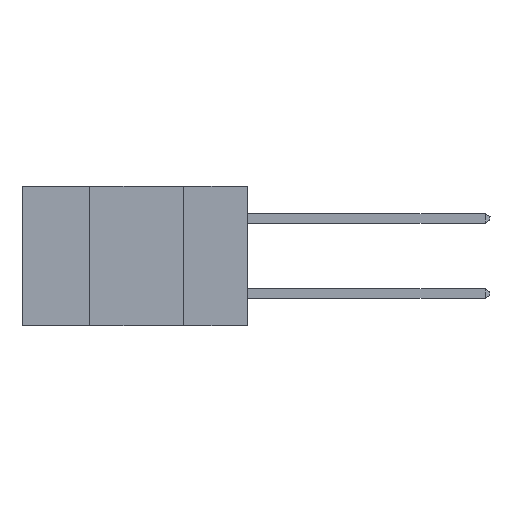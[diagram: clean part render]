
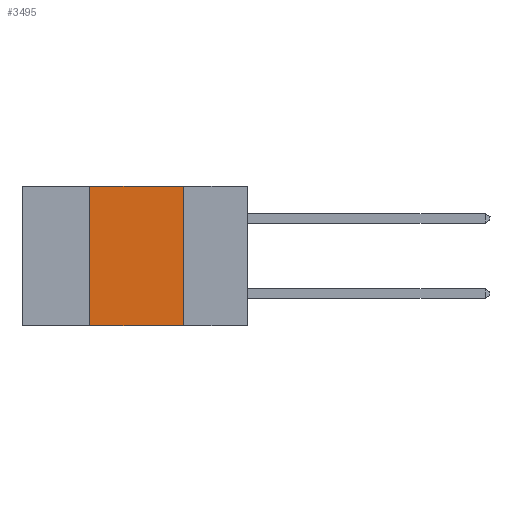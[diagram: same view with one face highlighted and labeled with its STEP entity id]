
A CAD part, left-side view. The second image highlights one B-rep face of the part: STEP entity #3495.
In plain terms, the highlighted planar face has unit normal (-1, 0, 0).
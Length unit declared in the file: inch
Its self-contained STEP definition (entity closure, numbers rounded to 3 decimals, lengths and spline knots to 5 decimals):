
#65 = DIRECTION ( 'NONE',  ( 0., -1., 0. ) ) ;
#738 = DIRECTION ( 'NONE',  ( 0., -1., 0. ) ) ;
#1065 = EDGE_CURVE ( 'NONE', #9933, #8915, #4147, .T. ) ;
#1200 = ORIENTED_EDGE ( 'NONE', *, *, #1065, .F. ) ;
#2044 = VERTEX_POINT ( 'NONE', #11692 ) ;
#2107 = DIRECTION ( 'NONE',  ( 0., 0., -1. ) ) ;
#2259 = DIRECTION ( 'NONE',  ( 0., 0., 1. ) ) ;
#2519 = LINE ( 'NONE', #5392, #11917 ) ;
#2683 = ORIENTED_EDGE ( 'NONE', *, *, #5785, .F. ) ;
#2806 = PLANE ( 'NONE',  #11710 ) ;
#3495 = ADVANCED_FACE ( 'NONE', ( #6768 ), #2806, .F. ) ;
#3760 = CARTESIAN_POINT ( 'NONE',  ( 0., 0.6, 0. ) ) ;
#3785 = LINE ( 'NONE', #6608, #6334 ) ;
#4147 = LINE ( 'NONE', #4269, #9241 ) ;
#4269 = CARTESIAN_POINT ( 'NONE',  ( 0., 0.42, -0.37 ) ) ;
#4533 = CARTESIAN_POINT ( 'NONE',  ( 0., 0.17, -0.37 ) ) ;
#4621 = CARTESIAN_POINT ( 'NONE',  ( 0., 0.42, -0.37 ) ) ;
#5392 = CARTESIAN_POINT ( 'NONE',  ( 0., 0.6, -0.37 ) ) ;
#5571 = ORIENTED_EDGE ( 'NONE', *, *, #12126, .T. ) ;
#5689 = CARTESIAN_POINT ( 'NONE',  ( 0., 0.17, -0.37 ) ) ;
#5704 = EDGE_CURVE ( 'NONE', #8915, #2044, #3785, .T. ) ;
#5785 = EDGE_CURVE ( 'NONE', #2044, #12057, #10746, .T. ) ;
#5986 = ORIENTED_EDGE ( 'NONE', *, *, #5704, .F. ) ;
#6287 = EDGE_LOOP ( 'NONE', ( #2683, #5986, #1200, #5571 ) ) ;
#6334 = VECTOR ( 'NONE', #65, 39.37008 ) ;
#6581 = DIRECTION ( 'NONE',  ( 0., 0., -1. ) ) ;
#6608 = CARTESIAN_POINT ( 'NONE',  ( 0., 0.6, 0. ) ) ;
#6768 = FACE_OUTER_BOUND ( 'NONE', #6287, .T. ) ;
#7656 = DIRECTION ( 'NONE',  ( 1., 0., 0. ) ) ;
#8372 = VECTOR ( 'NONE', #2107, 39.37008 ) ;
#8915 = VERTEX_POINT ( 'NONE', #12344 ) ;
#9241 = VECTOR ( 'NONE', #2259, 39.37008 ) ;
#9933 = VERTEX_POINT ( 'NONE', #4621 ) ;
#10746 = LINE ( 'NONE', #5689, #8372 ) ;
#11692 = CARTESIAN_POINT ( 'NONE',  ( 0., 0.17, 0. ) ) ;
#11710 = AXIS2_PLACEMENT_3D ( 'NONE', #3760, #7656, #6581 ) ;
#11917 = VECTOR ( 'NONE', #738, 39.37008 ) ;
#12057 = VERTEX_POINT ( 'NONE', #4533 ) ;
#12126 = EDGE_CURVE ( 'NONE', #9933, #12057, #2519, .T. ) ;
#12344 = CARTESIAN_POINT ( 'NONE',  ( 0., 0.42, 0. ) ) ;
